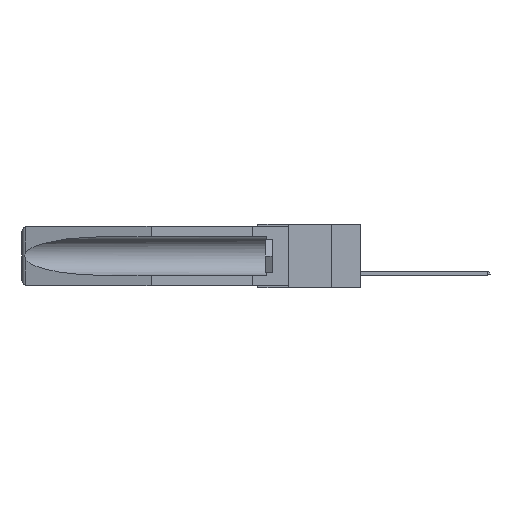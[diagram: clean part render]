
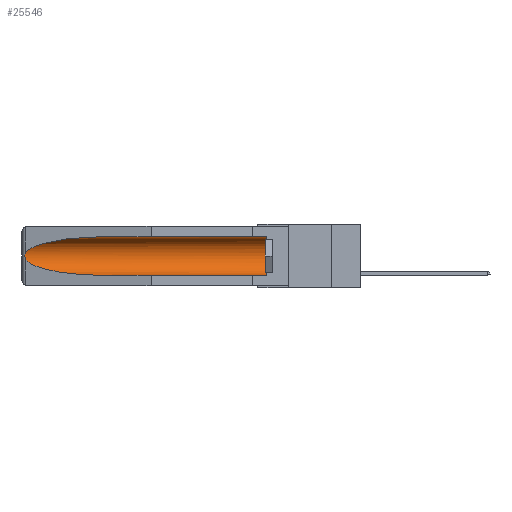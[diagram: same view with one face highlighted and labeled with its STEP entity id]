
A CAD part, left-side view. The second image highlights one B-rep face of the part: STEP entity #25546.
In plain terms, the highlighted cylindrical face has radius 2.857 mm (diameter 5.715 mm), a partial arc.
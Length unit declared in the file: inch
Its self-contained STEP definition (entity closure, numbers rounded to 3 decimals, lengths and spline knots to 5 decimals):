
#394 = VERTEX_POINT ( 'NONE', #24860 ) ;
#549 = CARTESIAN_POINT ( 'NONE',  ( 0.155, 1.07973, -0.284 ) ) ;
#674 = EDGE_CURVE ( 'NONE', #20459, #6702, #1377, .T. ) ;
#776 = CARTESIAN_POINT ( 'NONE',  ( 0.25451, 1.48313, -0.09465 ) ) ;
#1377 =( BOUNDED_CURVE ( )  B_SPLINE_CURVE ( 3, ( #29135, #6337, #776, #21271 ),
 .UNSPECIFIED., .F., .F. ) 
 B_SPLINE_CURVE_WITH_KNOTS ( ( 4, 4 ),
 ( 4.71239, 6.08839 ),
 .UNSPECIFIED. ) 
 CURVE ( )  GEOMETRIC_REPRESENTATION_ITEM ( )  RATIONAL_B_SPLINE_CURVE ( ( 1., 0.848, 0.848, 1. ) ) 
 REPRESENTATION_ITEM ( '' )  );
#1881 = CARTESIAN_POINT ( 'NONE',  ( 0.25451, 1.48313, -0.24835 ) ) ;
#1915 = CARTESIAN_POINT ( 'NONE',  ( 0.155, -0.30754, -0.059 ) ) ;
#3048 = EDGE_CURVE ( 'NONE', #394, #3664, #33114, .T. ) ;
#3121 = CARTESIAN_POINT ( 'NONE',  ( 0.26537, 1.52718, -0.14972 ) ) ;
#3447 = DIRECTION ( 'NONE',  ( 0., 1., 0. ) ) ;
#3664 = VERTEX_POINT ( 'NONE', #549 ) ;
#3767 = DIRECTION ( 'NONE',  ( 0., 0., 1. ) ) ;
#4256 = B_SPLINE_CURVE_WITH_KNOTS ( 'NONE', 3,
 ( #10430, #23443, #7727, #18414, #13024, #20639, #10540, #8060, #23335, #26061 ),
 .UNSPECIFIED., .F., .F.,
 ( 4, 2, 2, 2, 4 ),
 ( 0., 0.00029, 0.00058, 0.00087, 0.00117 ),
 .UNSPECIFIED. ) ;
#5017 = EDGE_CURVE ( 'NONE', #394, #33173, #11716, .T. ) ;
#5496 = CARTESIAN_POINT ( 'NONE',  ( 0.155, -0.30754, -0.284 ) ) ;
#6337 = CARTESIAN_POINT ( 'NONE',  ( 0.21114, 1.30732, -0.059 ) ) ;
#6702 = VERTEX_POINT ( 'NONE', #3121 ) ;
#7292 = EDGE_CURVE ( 'NONE', #33173, #20459, #24083, .T. ) ;
#7727 = CARTESIAN_POINT ( 'NONE',  ( 0.26654, 1.53092, -0.15636 ) ) ;
#7779 = ORIENTED_EDGE ( 'NONE', *, *, #21561, .T. ) ;
#8060 = CARTESIAN_POINT ( 'NONE',  ( 0.26655, 1.53094, -0.18657 ) ) ;
#8926 = CARTESIAN_POINT ( 'NONE',  ( 0.155, 0.126, -0.1715 ) ) ;
#9044 = DIRECTION ( 'NONE',  ( 0., -1., 0. ) ) ;
#9619 = CARTESIAN_POINT ( 'NONE',  ( 0.21114, 1.30732, -0.284 ) ) ;
#10120 = CYLINDRICAL_SURFACE ( 'NONE', #16595, 0.1125 ) ;
#10286 = CARTESIAN_POINT ( 'NONE',  ( 0.155, 0.126, -0.059 ) ) ;
#10430 = CARTESIAN_POINT ( 'NONE',  ( 0.26537, 1.52718, -0.14972 ) ) ;
#10540 = CARTESIAN_POINT ( 'NONE',  ( 0.2673, 1.53269, -0.17917 ) ) ;
#11716 = CIRCLE ( 'NONE', #30233, 0.1125 ) ;
#12277 = CARTESIAN_POINT ( 'NONE',  ( 0.155, 1.07973, -0.059 ) ) ;
#12372 = DIRECTION ( 'NONE',  ( 0., 1., 0. ) ) ;
#13024 = CARTESIAN_POINT ( 'NONE',  ( 0.2675, 1.53308, -0.16763 ) ) ;
#13345 =( BOUNDED_CURVE ( )  B_SPLINE_CURVE ( 3, ( #27724, #1881, #9619, #32501 ),
 .UNSPECIFIED., .F., .F. ) 
 B_SPLINE_CURVE_WITH_KNOTS ( ( 4, 4 ),
 ( 0.1948, 1.5708 ),
 .UNSPECIFIED. ) 
 CURVE ( )  GEOMETRIC_REPRESENTATION_ITEM ( )  RATIONAL_B_SPLINE_CURVE ( ( 1., 0.848, 0.848, 1. ) ) 
 REPRESENTATION_ITEM ( '' )  );
#15861 = CARTESIAN_POINT ( 'NONE',  ( 0.26537, 1.52718, -0.19328 ) ) ;
#15894 = ORIENTED_EDGE ( 'NONE', *, *, #674, .T. ) ;
#16595 = AXIS2_PLACEMENT_3D ( 'NONE', #31022, #31341, #28560 ) ;
#17768 = FACE_OUTER_BOUND ( 'NONE', #25605, .T. ) ;
#18414 = CARTESIAN_POINT ( 'NONE',  ( 0.2673, 1.5327, -0.16383 ) ) ;
#19647 = ORIENTED_EDGE ( 'NONE', *, *, #7292, .T. ) ;
#20459 = VERTEX_POINT ( 'NONE', #12277 ) ;
#20639 = CARTESIAN_POINT ( 'NONE',  ( 0.2675, 1.53308, -0.17534 ) ) ;
#21271 = CARTESIAN_POINT ( 'NONE',  ( 0.26537, 1.52718, -0.14972 ) ) ;
#21561 = EDGE_CURVE ( 'NONE', #6702, #30527, #4256, .T. ) ;
#22916 = EDGE_CURVE ( 'NONE', #30527, #3664, #13345, .T. ) ;
#23335 = CARTESIAN_POINT ( 'NONE',  ( 0.26597, 1.5296, -0.19026 ) ) ;
#23443 = CARTESIAN_POINT ( 'NONE',  ( 0.26597, 1.52961, -0.15275 ) ) ;
#24083 = LINE ( 'NONE', #1915, #30110 ) ;
#24860 = CARTESIAN_POINT ( 'NONE',  ( 0.155, 0.126, -0.284 ) ) ;
#25546 = ADVANCED_FACE ( 'NONE', ( #17768 ), #10120, .F. ) ;
#25605 = EDGE_LOOP ( 'NONE', ( #15894, #7779, #31258, #27196, #29286, #19647 ) ) ;
#26061 = CARTESIAN_POINT ( 'NONE',  ( 0.26537, 1.52718, -0.19328 ) ) ;
#27196 = ORIENTED_EDGE ( 'NONE', *, *, #3048, .F. ) ;
#27724 = CARTESIAN_POINT ( 'NONE',  ( 0.26537, 1.52718, -0.19328 ) ) ;
#28560 = DIRECTION ( 'NONE',  ( 0., 0., 1. ) ) ;
#29135 = CARTESIAN_POINT ( 'NONE',  ( 0.155, 1.07973, -0.059 ) ) ;
#29286 = ORIENTED_EDGE ( 'NONE', *, *, #5017, .T. ) ;
#30110 = VECTOR ( 'NONE', #12372, 39.37008 ) ;
#30233 = AXIS2_PLACEMENT_3D ( 'NONE', #8926, #9044, #3767 ) ;
#30527 = VERTEX_POINT ( 'NONE', #15861 ) ;
#31022 = CARTESIAN_POINT ( 'NONE',  ( 0.155, -0.30754, -0.1715 ) ) ;
#31258 = ORIENTED_EDGE ( 'NONE', *, *, #22916, .T. ) ;
#31341 = DIRECTION ( 'NONE',  ( 0., 1., 0. ) ) ;
#32317 = VECTOR ( 'NONE', #3447, 39.37008 ) ;
#32501 = CARTESIAN_POINT ( 'NONE',  ( 0.155, 1.07973, -0.284 ) ) ;
#33114 = LINE ( 'NONE', #5496, #32317 ) ;
#33173 = VERTEX_POINT ( 'NONE', #10286 ) ;
